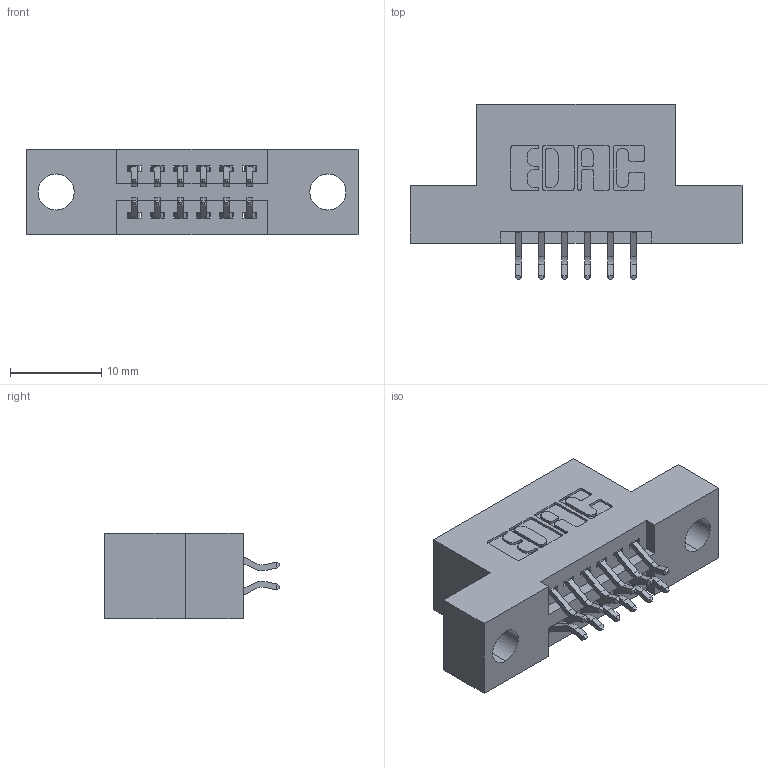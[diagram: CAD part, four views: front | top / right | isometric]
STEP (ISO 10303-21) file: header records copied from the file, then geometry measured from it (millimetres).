
FILE_DESCRIPTION (( 'STEP AP203' ), '1' );
FILE_NAME ('395-012-556-204.STEP', '2018-11-05T19:37:14', ( '' ), ( '' ), 'SwSTEP 2.0', 'SolidWorks 2016', '' );
FILE_SCHEMA (( 'CONFIG_CONTROL_DESIGN' ));
Length unit declared in the file: inch
Products named in the file (3): 345 Part_Flush Mounting Lugs - 0.156 Dia-TH; 345-292-001_556 Tail; 395-012-556-204
Assembly tree (13 placements, depth 2):
  395-012-556-204
    345 Part_Flush Mounting Lugs - 0.156 Dia-TH
    345-292-001_556 Tail  x12
Bounding box: 36.45 x 19.24 x 9.4 mm (x, y, z)
Volume: 3118.2 mm3; surface area: 3716.6 mm2
Topology: 13 solids, 13 shells, 798 faces, 2345 edges, 1546 vertices
Faces by surface type: plane 524, cylinder 274
Entity records: 9777 total; most frequent: CARTESIAN_POINT 1688, ORIENTED_EDGE 1610, DIRECTION 1521, EDGE_CURVE 805, VECTOR 641, LINE 641, VERTEX_POINT 534, AXIS2_PLACEMENT_3D 440
